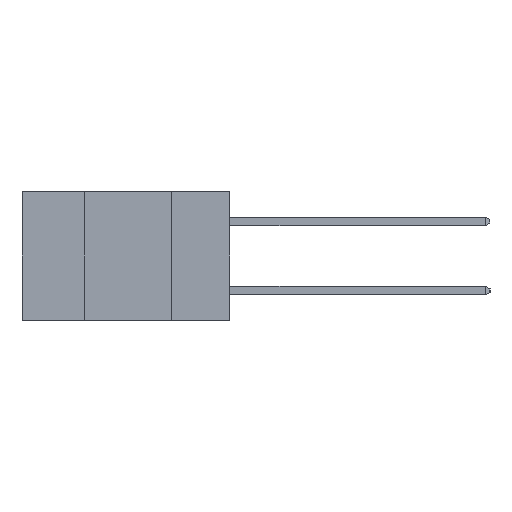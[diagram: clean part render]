
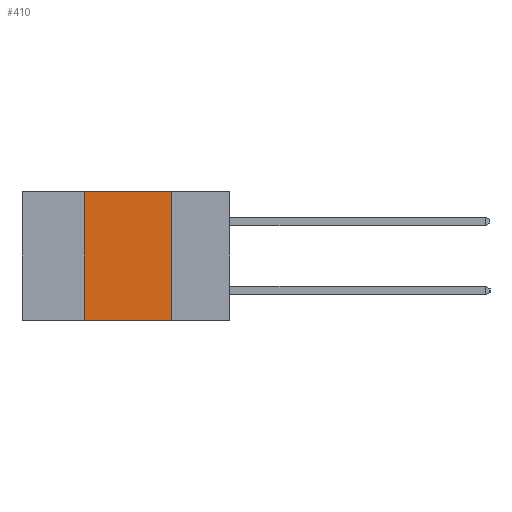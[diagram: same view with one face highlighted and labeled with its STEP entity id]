
A CAD part, left-side view. The second image highlights one B-rep face of the part: STEP entity #410.
In plain terms, the highlighted planar face has unit normal (-1, 0, 0).
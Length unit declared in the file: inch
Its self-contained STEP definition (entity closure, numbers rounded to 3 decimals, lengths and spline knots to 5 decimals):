
#295 = DIRECTION ( 'NONE',  ( 1., 0., 0. ) ) ;
#349 = DIRECTION ( 'NONE',  ( 0., 0., -1. ) ) ;
#410 = ADVANCED_FACE ( 'NONE', ( #4107 ), #2126, .F. ) ;
#1247 = CARTESIAN_POINT ( 'NONE',  ( 0., 0.42, -0.37 ) ) ;
#1366 = VECTOR ( 'NONE', #10225, 39.37008 ) ;
#1473 = EDGE_CURVE ( 'NONE', #4680, #10144, #10383, .T. ) ;
#2126 = PLANE ( 'NONE',  #14560 ) ;
#3601 = ORIENTED_EDGE ( 'NONE', *, *, #10609, .F. ) ;
#3935 = ORIENTED_EDGE ( 'NONE', *, *, #6848, .F. ) ;
#4107 = FACE_OUTER_BOUND ( 'NONE', #14065, .T. ) ;
#4264 = ORIENTED_EDGE ( 'NONE', *, *, #4548, .T. ) ;
#4390 = DIRECTION ( 'NONE',  ( 0., 0., -1. ) ) ;
#4420 = CARTESIAN_POINT ( 'NONE',  ( 0., 0.17, -0.37 ) ) ;
#4548 = EDGE_CURVE ( 'NONE', #14585, #5297, #10171, .T. ) ;
#4680 = VERTEX_POINT ( 'NONE', #6634 ) ;
#5297 = VERTEX_POINT ( 'NONE', #11080 ) ;
#6634 = CARTESIAN_POINT ( 'NONE',  ( 0., 0.42, 0. ) ) ;
#6848 = EDGE_CURVE ( 'NONE', #14585, #4680, #14254, .T. ) ;
#7340 = CARTESIAN_POINT ( 'NONE',  ( 0., 0.17, 0. ) ) ;
#9007 = CARTESIAN_POINT ( 'NONE',  ( 0., 0.42, -0.37 ) ) ;
#9037 = DIRECTION ( 'NONE',  ( 0., 0., 1. ) ) ;
#9865 = CARTESIAN_POINT ( 'NONE',  ( 0., 0.6, -0.37 ) ) ;
#10144 = VERTEX_POINT ( 'NONE', #7340 ) ;
#10171 = LINE ( 'NONE', #9865, #12794 ) ;
#10225 = DIRECTION ( 'NONE',  ( 0., -1., 0. ) ) ;
#10262 = CARTESIAN_POINT ( 'NONE',  ( 0., 0.6, 0. ) ) ;
#10383 = LINE ( 'NONE', #10262, #1366 ) ;
#10609 = EDGE_CURVE ( 'NONE', #10144, #5297, #13828, .T. ) ;
#10874 = CARTESIAN_POINT ( 'NONE',  ( 0., 0.6, 0. ) ) ;
#10998 = VECTOR ( 'NONE', #9037, 39.37008 ) ;
#11080 = CARTESIAN_POINT ( 'NONE',  ( 0., 0.17, -0.37 ) ) ;
#12505 = ORIENTED_EDGE ( 'NONE', *, *, #1473, .F. ) ;
#12794 = VECTOR ( 'NONE', #13015, 39.37008 ) ;
#13015 = DIRECTION ( 'NONE',  ( 0., -1., 0. ) ) ;
#13496 = VECTOR ( 'NONE', #4390, 39.37008 ) ;
#13828 = LINE ( 'NONE', #4420, #13496 ) ;
#14065 = EDGE_LOOP ( 'NONE', ( #3601, #12505, #3935, #4264 ) ) ;
#14254 = LINE ( 'NONE', #9007, #10998 ) ;
#14560 = AXIS2_PLACEMENT_3D ( 'NONE', #10874, #295, #349 ) ;
#14585 = VERTEX_POINT ( 'NONE', #1247 ) ;
